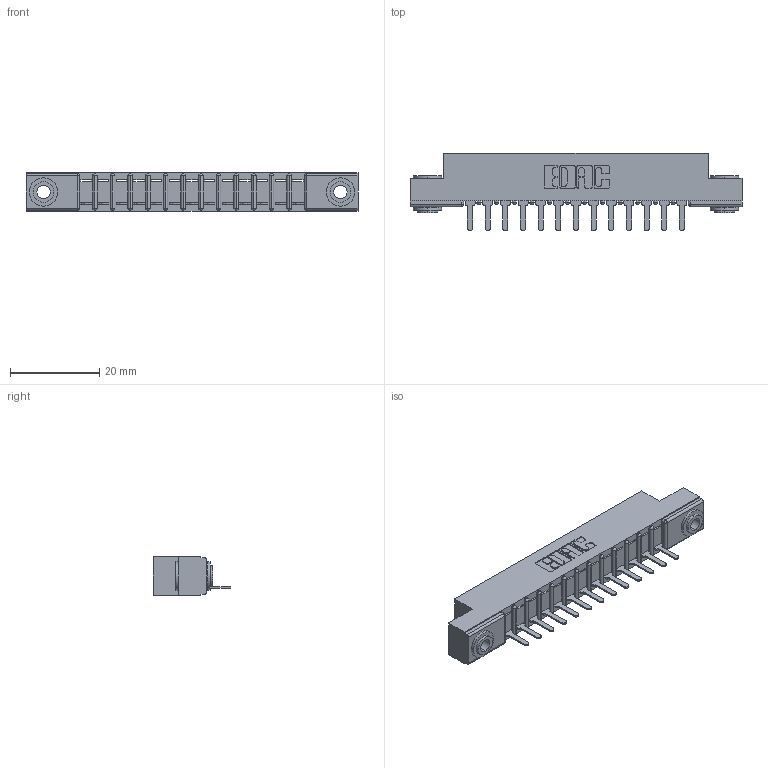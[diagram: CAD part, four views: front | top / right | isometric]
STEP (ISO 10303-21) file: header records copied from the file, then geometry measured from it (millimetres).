
FILE_DESCRIPTION (( 'STEP AP203' ), '1' );
FILE_NAME ('307-013-425-103.STEP', '2020-09-25T12:47:55', ( '' ), ( '' ), 'SwSTEP 2.0', 'SolidWorks 2020', '' );
FILE_SCHEMA (( 'CONFIG_CONTROL_DESIGN' ));
Length unit declared in the file: inch
Products named in the file (7): 307-013-425-103; 307 Part_.156 Dia Mounting Holes; 345-250-002_345-250-002-102; 307-290-001_525; 307-013-425-104
Assembly tree (16 placements, depth 2):
  307-013-425-103
    307 Part_.156 Dia Mounting Holes
    307-290-001_525  x13
    345-250-002_345-250-002-102  x2
  307 Part_.156 Dia Mounting Holes
  307-290-001_525
  307-013-425-104
Bounding box: 74.52 x 17.42 x 8.71 mm (x, y, z)
Volume: 4718.8 mm3; surface area: 7158 mm2
Topology: 16 solids, 16 shells, 912 faces, 2541 edges, 1634 vertices
Faces by surface type: plane 575, cylinder 301, sphere 28, cone 8
Entity records: 37114 total; most frequent: CARTESIAN_POINT 6200, ORIENTED_EDGE 6118, DIRECTION 6020, EDGE_CURVE 3076, LINE 2367, VECTOR 2316, VERTEX_POINT 1994, AXIS2_PLACEMENT_3D 1884
